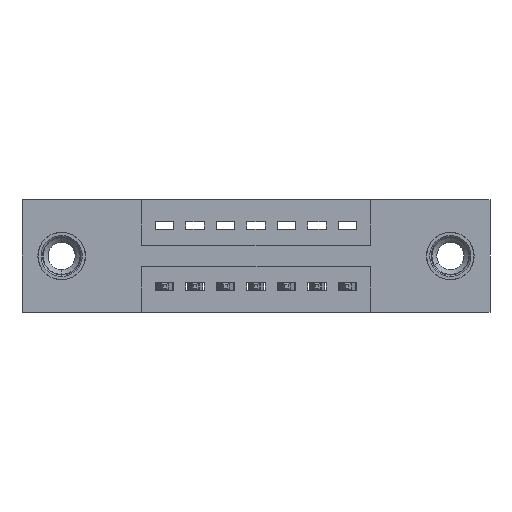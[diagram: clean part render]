
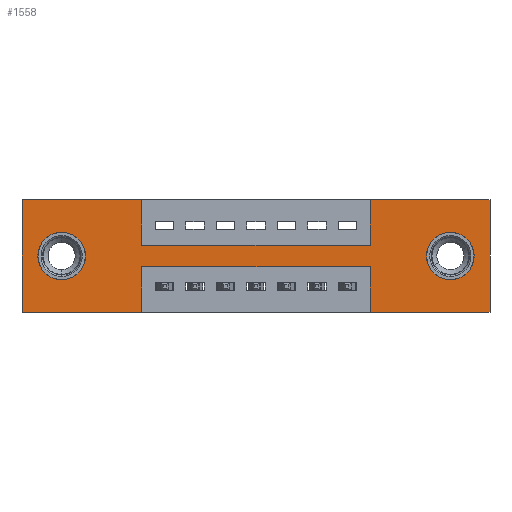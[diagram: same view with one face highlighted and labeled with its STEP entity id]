
A CAD part, front view. The second image highlights one B-rep face of the part: STEP entity #1558.
In plain terms, the highlighted planar face has unit normal (0, -1, 0).
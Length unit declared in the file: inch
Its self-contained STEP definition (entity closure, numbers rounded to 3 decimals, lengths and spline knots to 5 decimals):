
#18 = CIRCLE ( 'NONE', #7274, 0.078 ) ;
#232 = VECTOR ( 'NONE', #3080, 39.37008 ) ;
#313 = DIRECTION ( 'NONE',  ( 0., 0., -1. ) ) ;
#435 = VERTEX_POINT ( 'NONE', #1441 ) ;
#568 = DIRECTION ( 'NONE',  ( 0., -1., 0. ) ) ;
#699 = CARTESIAN_POINT ( 'NONE',  ( 1.1425, 0., -0.15 ) ) ;
#775 = CARTESIAN_POINT ( 'NONE',  ( 0.3925, 0., -0.37 ) ) ;
#807 = VECTOR ( 'NONE', #8229, 39.37008 ) ;
#936 = VECTOR ( 'NONE', #10243, 39.37008 ) ;
#977 = DIRECTION ( 'NONE',  ( 1., 0., 0. ) ) ;
#982 = LINE ( 'NONE', #7674, #5827 ) ;
#1000 = ORIENTED_EDGE ( 'NONE', *, *, #7960, .T. ) ;
#1095 = DIRECTION ( 'NONE',  ( 0., 1., 0. ) ) ;
#1278 = ORIENTED_EDGE ( 'NONE', *, *, #6389, .T. ) ;
#1334 = VERTEX_POINT ( 'NONE', #10523 ) ;
#1441 = CARTESIAN_POINT ( 'NONE',  ( 1.1425, 0., -0.37 ) ) ;
#1450 = VECTOR ( 'NONE', #4256, 39.37008 ) ;
#1539 = LINE ( 'NONE', #4443, #8301 ) ;
#1558 = ADVANCED_FACE ( 'NONE', ( #8775, #9028, #4521 ), #9798, .T. ) ;
#1610 = EDGE_LOOP ( 'NONE', ( #4688, #4986, #3766, #6822, #6725, #2999, #6068, #3695, #4693, #6212, #9927, #6504 ) ) ;
#1656 = CARTESIAN_POINT ( 'NONE',  ( 0., 0., -0.37 ) ) ;
#1725 = CARTESIAN_POINT ( 'NONE',  ( 0., 0., 0. ) ) ;
#1838 = EDGE_CURVE ( 'NONE', #9023, #4113, #8013, .T. ) ;
#1863 = CARTESIAN_POINT ( 'NONE',  ( 0.13, 0., -0.185 ) ) ;
#2062 = CARTESIAN_POINT ( 'NONE',  ( 0., 0., 0. ) ) ;
#2166 = LINE ( 'NONE', #8306, #232 ) ;
#2226 = EDGE_CURVE ( 'NONE', #7599, #4274, #4648, .T. ) ;
#2402 = DIRECTION ( 'NONE',  ( -1., 0., 0. ) ) ;
#2611 = DIRECTION ( 'NONE',  ( 0., 0., -1. ) ) ;
#2632 = CARTESIAN_POINT ( 'NONE',  ( 0.13, 0., -0.185 ) ) ;
#2785 = DIRECTION ( 'NONE',  ( 0., 0., 1. ) ) ;
#2999 = ORIENTED_EDGE ( 'NONE', *, *, #7060, .F. ) ;
#3034 = CARTESIAN_POINT ( 'NONE',  ( 1.405, 0., -0.185 ) ) ;
#3080 = DIRECTION ( 'NONE',  ( -1., 0., 0. ) ) ;
#3282 = EDGE_CURVE ( 'NONE', #7038, #1334, #8273, .T. ) ;
#3340 = CARTESIAN_POINT ( 'NONE',  ( 0.13, 0., -0.107 ) ) ;
#3442 = CARTESIAN_POINT ( 'NONE',  ( 1.1425, 0., -0.22 ) ) ;
#3487 = ORIENTED_EDGE ( 'NONE', *, *, #3282, .T. ) ;
#3540 = DIRECTION ( 'NONE',  ( 0., 0., 1. ) ) ;
#3695 = ORIENTED_EDGE ( 'NONE', *, *, #6053, .F. ) ;
#3766 = ORIENTED_EDGE ( 'NONE', *, *, #9043, .F. ) ;
#4004 = LINE ( 'NONE', #10071, #10418 ) ;
#4113 = VERTEX_POINT ( 'NONE', #10553 ) ;
#4132 = CIRCLE ( 'NONE', #4192, 0.078 ) ;
#4164 = LINE ( 'NONE', #10897, #1450 ) ;
#4192 = AXIS2_PLACEMENT_3D ( 'NONE', #2632, #8684, #3540 ) ;
#4256 = DIRECTION ( 'NONE',  ( 0., 0., -1. ) ) ;
#4274 = VERTEX_POINT ( 'NONE', #10323 ) ;
#4437 = VECTOR ( 'NONE', #7019, 39.37008 ) ;
#4438 = VERTEX_POINT ( 'NONE', #9299 ) ;
#4443 = CARTESIAN_POINT ( 'NONE',  ( 0.3925, 0., -0.22 ) ) ;
#4473 = VERTEX_POINT ( 'NONE', #3340 ) ;
#4521 = FACE_OUTER_BOUND ( 'NONE', #1610, .T. ) ;
#4644 = CARTESIAN_POINT ( 'NONE',  ( 0.3925, 0., -0.15 ) ) ;
#4646 = CARTESIAN_POINT ( 'NONE',  ( 0.13, 0., -0.263 ) ) ;
#4648 = LINE ( 'NONE', #5798, #10962 ) ;
#4688 = ORIENTED_EDGE ( 'NONE', *, *, #5082, .F. ) ;
#4693 = ORIENTED_EDGE ( 'NONE', *, *, #9897, .F. ) ;
#4986 = ORIENTED_EDGE ( 'NONE', *, *, #7406, .F. ) ;
#5082 = EDGE_CURVE ( 'NONE', #6420, #9078, #4164, .T. ) ;
#5104 = CARTESIAN_POINT ( 'NONE',  ( 1.535, 0., 0. ) ) ;
#5120 = VECTOR ( 'NONE', #977, 39.37008 ) ;
#5270 = CARTESIAN_POINT ( 'NONE',  ( 1.405, 0., -0.107 ) ) ;
#5418 = CARTESIAN_POINT ( 'NONE',  ( 1.405, 0., -0.185 ) ) ;
#5635 = VECTOR ( 'NONE', #9335, 39.37008 ) ;
#5656 = CARTESIAN_POINT ( 'NONE',  ( 0.3925, 0., 0. ) ) ;
#5741 = EDGE_CURVE ( 'NONE', #9863, #7599, #4004, .T. ) ;
#5798 = CARTESIAN_POINT ( 'NONE',  ( 0., 0., 0. ) ) ;
#5827 = VECTOR ( 'NONE', #2402, 39.37008 ) ;
#5989 = EDGE_LOOP ( 'NONE', ( #3487, #10605 ) ) ;
#6053 = EDGE_CURVE ( 'NONE', #11208, #9023, #7423, .T. ) ;
#6068 = ORIENTED_EDGE ( 'NONE', *, *, #1838, .F. ) ;
#6146 = CARTESIAN_POINT ( 'NONE',  ( 1.1425, 0., -0.37 ) ) ;
#6212 = ORIENTED_EDGE ( 'NONE', *, *, #2226, .F. ) ;
#6229 = CARTESIAN_POINT ( 'NONE',  ( 1.535, 0., 0. ) ) ;
#6246 = CARTESIAN_POINT ( 'NONE',  ( 0.3925, 0., -0.22 ) ) ;
#6255 = DIRECTION ( 'NONE',  ( -1., 0., 0. ) ) ;
#6311 = DIRECTION ( 'NONE',  ( 0., 0., -1. ) ) ;
#6389 = EDGE_CURVE ( 'NONE', #4473, #10661, #4132, .T. ) ;
#6420 = VERTEX_POINT ( 'NONE', #6246 ) ;
#6447 = VECTOR ( 'NONE', #8199, 39.37008 ) ;
#6504 = ORIENTED_EDGE ( 'NONE', *, *, #8174, .F. ) ;
#6725 = ORIENTED_EDGE ( 'NONE', *, *, #7262, .F. ) ;
#6822 = ORIENTED_EDGE ( 'NONE', *, *, #8901, .F. ) ;
#6898 = AXIS2_PLACEMENT_3D ( 'NONE', #1656, #568, #313 ) ;
#7019 = DIRECTION ( 'NONE',  ( 0., 0., 1. ) ) ;
#7038 = VERTEX_POINT ( 'NONE', #5270 ) ;
#7060 = EDGE_CURVE ( 'NONE', #4113, #8471, #7794, .T. ) ;
#7120 = EDGE_CURVE ( 'NONE', #1334, #7038, #18, .T. ) ;
#7141 = CARTESIAN_POINT ( 'NONE',  ( 0.3925, 0., -0.15 ) ) ;
#7240 = DIRECTION ( 'NONE',  ( 1., 0., 0. ) ) ;
#7262 = EDGE_CURVE ( 'NONE', #8471, #4438, #8178, .T. ) ;
#7274 = AXIS2_PLACEMENT_3D ( 'NONE', #5418, #11133, #6311 ) ;
#7406 = EDGE_CURVE ( 'NONE', #8394, #6420, #1539, .T. ) ;
#7423 = LINE ( 'NONE', #4644, #5120 ) ;
#7461 = CARTESIAN_POINT ( 'NONE',  ( 1.1425, 0., 0. ) ) ;
#7599 = VERTEX_POINT ( 'NONE', #2062 ) ;
#7674 = CARTESIAN_POINT ( 'NONE',  ( 0., 0., -0.37 ) ) ;
#7794 = LINE ( 'NONE', #1725, #936 ) ;
#7936 = LINE ( 'NONE', #5656, #807 ) ;
#7960 = EDGE_CURVE ( 'NONE', #10661, #4473, #11030, .T. ) ;
#8013 = LINE ( 'NONE', #7461, #6447 ) ;
#8034 = DIRECTION ( 'NONE',  ( 0., 1., 0. ) ) ;
#8163 = CARTESIAN_POINT ( 'NONE',  ( 0., 0., -0.37 ) ) ;
#8174 = EDGE_CURVE ( 'NONE', #9078, #9863, #2166, .T. ) ;
#8178 = LINE ( 'NONE', #5104, #5635 ) ;
#8199 = DIRECTION ( 'NONE',  ( 0., 0., 1. ) ) ;
#8229 = DIRECTION ( 'NONE',  ( 0., 0., -1. ) ) ;
#8273 = CIRCLE ( 'NONE', #8615, 0.078 ) ;
#8301 = VECTOR ( 'NONE', #6255, 39.37008 ) ;
#8306 = CARTESIAN_POINT ( 'NONE',  ( 0., 0., -0.37 ) ) ;
#8327 = EDGE_LOOP ( 'NONE', ( #1278, #1000 ) ) ;
#8394 = VERTEX_POINT ( 'NONE', #3442 ) ;
#8471 = VERTEX_POINT ( 'NONE', #6229 ) ;
#8615 = AXIS2_PLACEMENT_3D ( 'NONE', #3034, #1095, #2611 ) ;
#8684 = DIRECTION ( 'NONE',  ( 0., 1., 0. ) ) ;
#8775 = FACE_BOUND ( 'NONE', #5989, .T. ) ;
#8901 = EDGE_CURVE ( 'NONE', #4438, #435, #982, .T. ) ;
#9023 = VERTEX_POINT ( 'NONE', #699 ) ;
#9028 = FACE_BOUND ( 'NONE', #8327, .T. ) ;
#9043 = EDGE_CURVE ( 'NONE', #435, #8394, #10781, .T. ) ;
#9078 = VERTEX_POINT ( 'NONE', #775 ) ;
#9299 = CARTESIAN_POINT ( 'NONE',  ( 1.535, 0., -0.37 ) ) ;
#9335 = DIRECTION ( 'NONE',  ( 0., 0., -1. ) ) ;
#9798 = PLANE ( 'NONE',  #6898 ) ;
#9863 = VERTEX_POINT ( 'NONE', #8163 ) ;
#9897 = EDGE_CURVE ( 'NONE', #4274, #11208, #7936, .T. ) ;
#9927 = ORIENTED_EDGE ( 'NONE', *, *, #5741, .F. ) ;
#10071 = CARTESIAN_POINT ( 'NONE',  ( 0., 0., 0. ) ) ;
#10243 = DIRECTION ( 'NONE',  ( 1., 0., 0. ) ) ;
#10323 = CARTESIAN_POINT ( 'NONE',  ( 0.3925, 0., 0. ) ) ;
#10418 = VECTOR ( 'NONE', #10849, 39.37008 ) ;
#10523 = CARTESIAN_POINT ( 'NONE',  ( 1.405, 0., -0.263 ) ) ;
#10553 = CARTESIAN_POINT ( 'NONE',  ( 1.1425, 0., 0. ) ) ;
#10605 = ORIENTED_EDGE ( 'NONE', *, *, #7120, .T. ) ;
#10661 = VERTEX_POINT ( 'NONE', #4646 ) ;
#10781 = LINE ( 'NONE', #6146, #4437 ) ;
#10849 = DIRECTION ( 'NONE',  ( 0., 0., 1. ) ) ;
#10897 = CARTESIAN_POINT ( 'NONE',  ( 0.3925, 0., -0.37 ) ) ;
#10944 = AXIS2_PLACEMENT_3D ( 'NONE', #1863, #8034, #2785 ) ;
#10962 = VECTOR ( 'NONE', #7240, 39.37008 ) ;
#11030 = CIRCLE ( 'NONE', #10944, 0.078 ) ;
#11133 = DIRECTION ( 'NONE',  ( 0., 1., 0. ) ) ;
#11208 = VERTEX_POINT ( 'NONE', #7141 ) ;
